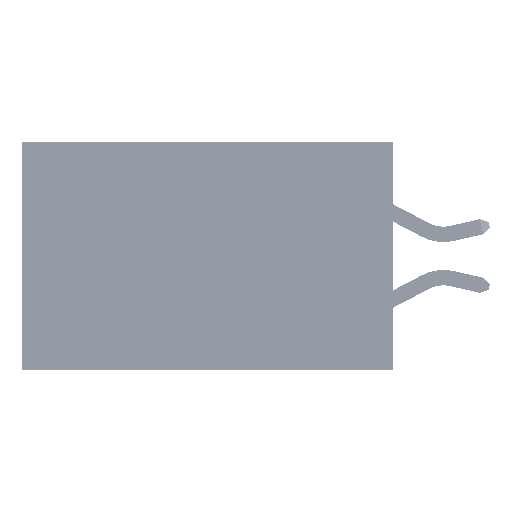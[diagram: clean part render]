
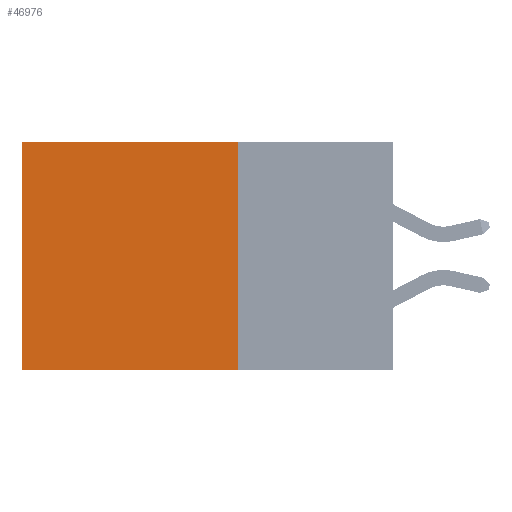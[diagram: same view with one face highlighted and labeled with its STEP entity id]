
A CAD part, left-side view. The second image highlights one B-rep face of the part: STEP entity #46976.
In plain terms, the highlighted planar face has unit normal (-1, 0, 0).
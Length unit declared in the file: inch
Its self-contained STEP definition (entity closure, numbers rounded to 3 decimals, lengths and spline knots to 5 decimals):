
#205 = DIRECTION ( 'NONE',  ( 0., 0., -1. ) ) ;
#1012 = VECTOR ( 'NONE', #41805, 39.37008 ) ;
#1606 = DIRECTION ( 'NONE',  ( 0., 0., -1. ) ) ;
#3577 = CARTESIAN_POINT ( 'NONE',  ( 0.2875, 0.25, 0. ) ) ;
#4425 = EDGE_CURVE ( 'NONE', #24215, #10104, #46163, .T. ) ;
#4524 = EDGE_CURVE ( 'NONE', #14833, #10005, #19857, .T. ) ;
#6935 = CARTESIAN_POINT ( 'NONE',  ( 0.2875, 0.6, -0.37 ) ) ;
#7218 = VECTOR ( 'NONE', #36982, 39.37008 ) ;
#7554 = FACE_OUTER_BOUND ( 'NONE', #45067, .T. ) ;
#8954 = CARTESIAN_POINT ( 'NONE',  ( 0.2875, 0.6, 0. ) ) ;
#9506 = VECTOR ( 'NONE', #205, 39.37008 ) ;
#10005 = VERTEX_POINT ( 'NONE', #6935 ) ;
#10104 = VERTEX_POINT ( 'NONE', #26785 ) ;
#13035 = ORIENTED_EDGE ( 'NONE', *, *, #42595, .T. ) ;
#14396 = VECTOR ( 'NONE', #45852, 39.37008 ) ;
#14833 = VERTEX_POINT ( 'NONE', #8954 ) ;
#17463 = EDGE_CURVE ( 'NONE', #10104, #10005, #27852, .T. ) ;
#19791 = CARTESIAN_POINT ( 'NONE',  ( 0.2875, 0.6, 0. ) ) ;
#19857 = LINE ( 'NONE', #19791, #9506 ) ;
#21130 = CARTESIAN_POINT ( 'NONE',  ( 0.2875, 0.25, 0. ) ) ;
#22622 = ORIENTED_EDGE ( 'NONE', *, *, #4425, .F. ) ;
#23037 = LINE ( 'NONE', #49273, #1012 ) ;
#24215 = VERTEX_POINT ( 'NONE', #24993 ) ;
#24993 = CARTESIAN_POINT ( 'NONE',  ( 0.2875, 0.25, 0. ) ) ;
#24995 = DIRECTION ( 'NONE',  ( 1., 0., 0. ) ) ;
#26785 = CARTESIAN_POINT ( 'NONE',  ( 0.2875, 0.25, -0.37 ) ) ;
#27852 = LINE ( 'NONE', #48316, #7218 ) ;
#32239 = AXIS2_PLACEMENT_3D ( 'NONE', #21130, #24995, #1606 ) ;
#34326 = ORIENTED_EDGE ( 'NONE', *, *, #17463, .F. ) ;
#36982 = DIRECTION ( 'NONE',  ( 0., 1., 0. ) ) ;
#40433 = ORIENTED_EDGE ( 'NONE', *, *, #4524, .T. ) ;
#41805 = DIRECTION ( 'NONE',  ( 0., 1., 0. ) ) ;
#42595 = EDGE_CURVE ( 'NONE', #24215, #14833, #23037, .T. ) ;
#43985 = PLANE ( 'NONE',  #32239 ) ;
#45067 = EDGE_LOOP ( 'NONE', ( #40433, #34326, #22622, #13035 ) ) ;
#45852 = DIRECTION ( 'NONE',  ( 0., 0., -1. ) ) ;
#46163 = LINE ( 'NONE', #3577, #14396 ) ;
#46976 = ADVANCED_FACE ( 'NONE', ( #7554 ), #43985, .F. ) ;
#48316 = CARTESIAN_POINT ( 'NONE',  ( 0.2875, 0.25, -0.37 ) ) ;
#49273 = CARTESIAN_POINT ( 'NONE',  ( 0.2875, 0.25, 0. ) ) ;
